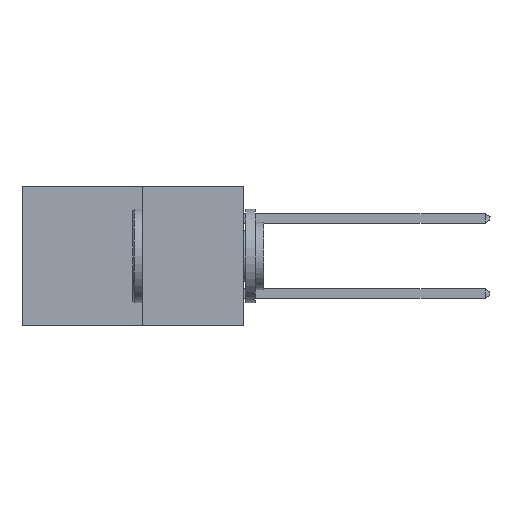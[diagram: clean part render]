
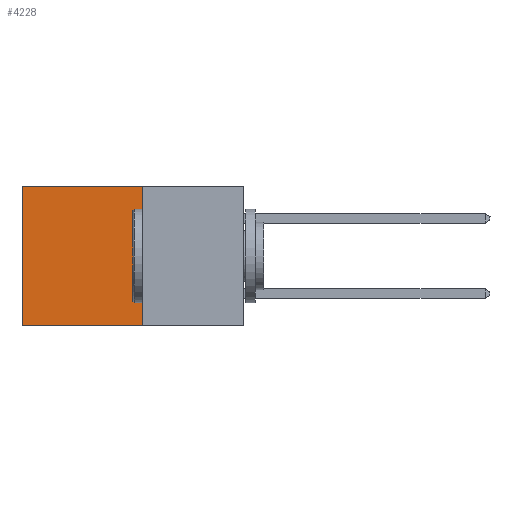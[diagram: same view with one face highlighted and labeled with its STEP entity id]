
A CAD part, left-side view. The second image highlights one B-rep face of the part: STEP entity #4228.
In plain terms, the highlighted planar face has unit normal (-1, 0, 0).
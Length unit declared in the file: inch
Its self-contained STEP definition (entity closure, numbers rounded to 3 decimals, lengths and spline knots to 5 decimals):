
#519 = LINE ( 'NONE', #3427, #4643 ) ;
#708 = EDGE_LOOP ( 'NONE', ( #5924, #9812, #1815, #3989 ) ) ;
#887 = AXIS2_PLACEMENT_3D ( 'NONE', #4819, #4787, #4785 ) ;
#937 = CARTESIAN_POINT ( 'NONE',  ( 0.277, 0.27, -0.37 ) ) ;
#1032 = DIRECTION ( 'NONE',  ( 0., 1., 0. ) ) ;
#1253 = VECTOR ( 'NONE', #1032, 39.37008 ) ;
#1686 = VECTOR ( 'NONE', #1788, 39.37008 ) ;
#1788 = DIRECTION ( 'NONE',  ( 0., 1., 0. ) ) ;
#1815 = ORIENTED_EDGE ( 'NONE', *, *, #5465, .F. ) ;
#2076 = CARTESIAN_POINT ( 'NONE',  ( 0.277, 0.27, 0. ) ) ;
#2366 = EDGE_CURVE ( 'NONE', #5582, #6640, #7858, .T. ) ;
#2416 = CARTESIAN_POINT ( 'NONE',  ( 0.277, 0.27, -0.37 ) ) ;
#2420 = DIRECTION ( 'NONE',  ( 0., 0., -1. ) ) ;
#3333 = CARTESIAN_POINT ( 'NONE',  ( 0.277, 0.27, 0. ) ) ;
#3427 = CARTESIAN_POINT ( 'NONE',  ( 0.277, 0.27, -0.37 ) ) ;
#3861 = LINE ( 'NONE', #2076, #1686 ) ;
#3880 = VECTOR ( 'NONE', #2420, 39.37008 ) ;
#3989 = ORIENTED_EDGE ( 'NONE', *, *, #5542, .T. ) ;
#3998 = CARTESIAN_POINT ( 'NONE',  ( 0.277, 0.59, -0.37 ) ) ;
#4027 = DIRECTION ( 'NONE',  ( 0., 0., -1. ) ) ;
#4228 = ADVANCED_FACE ( 'NONE', ( #4934 ), #4823, .F. ) ;
#4643 = VECTOR ( 'NONE', #4027, 39.37008 ) ;
#4785 = DIRECTION ( 'NONE',  ( 0., 0., -1. ) ) ;
#4787 = DIRECTION ( 'NONE',  ( 1., 0., 0. ) ) ;
#4819 = CARTESIAN_POINT ( 'NONE',  ( 0.277, 0.27, -0.37 ) ) ;
#4823 = PLANE ( 'NONE',  #887 ) ;
#4934 = FACE_OUTER_BOUND ( 'NONE', #708, .T. ) ;
#5464 = VERTEX_POINT ( 'NONE', #3333 ) ;
#5465 = EDGE_CURVE ( 'NONE', #5464, #5582, #519, .T. ) ;
#5542 = EDGE_CURVE ( 'NONE', #5464, #6420, #3861, .T. ) ;
#5582 = VERTEX_POINT ( 'NONE', #937 ) ;
#5924 = ORIENTED_EDGE ( 'NONE', *, *, #10008, .T. ) ;
#6060 = LINE ( 'NONE', #3998, #3880 ) ;
#6420 = VERTEX_POINT ( 'NONE', #7341 ) ;
#6640 = VERTEX_POINT ( 'NONE', #9681 ) ;
#7341 = CARTESIAN_POINT ( 'NONE',  ( 0.277, 0.59, 0. ) ) ;
#7858 = LINE ( 'NONE', #2416, #1253 ) ;
#9681 = CARTESIAN_POINT ( 'NONE',  ( 0.277, 0.59, -0.37 ) ) ;
#9812 = ORIENTED_EDGE ( 'NONE', *, *, #2366, .F. ) ;
#10008 = EDGE_CURVE ( 'NONE', #6420, #6640, #6060, .T. ) ;
